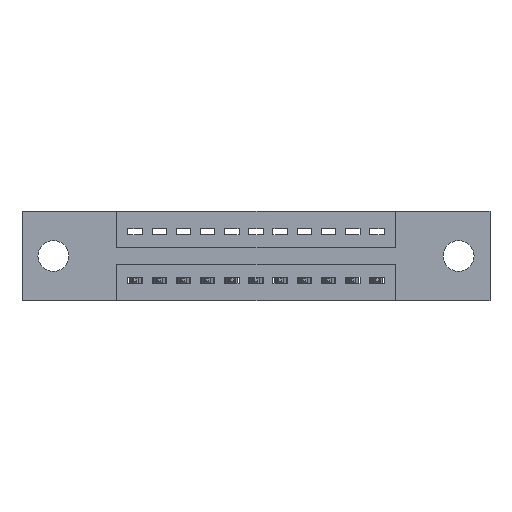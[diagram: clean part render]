
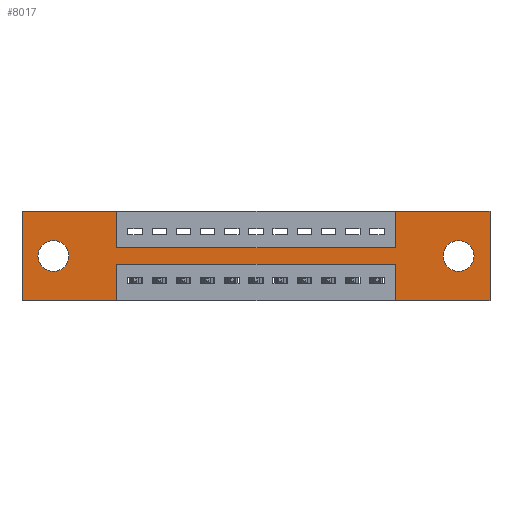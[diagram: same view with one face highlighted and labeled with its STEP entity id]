
A CAD part, front view. The second image highlights one B-rep face of the part: STEP entity #8017.
In plain terms, the highlighted planar face has unit normal (0, -1, 0).
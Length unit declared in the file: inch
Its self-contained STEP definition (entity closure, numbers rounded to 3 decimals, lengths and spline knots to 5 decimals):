
#35 = VERTEX_POINT ( 'NONE', #985 ) ;
#137 = EDGE_LOOP ( 'NONE', ( #1967, #1300 ) ) ;
#282 = EDGE_CURVE ( 'NONE', #7556, #35, #1522, .T. ) ;
#303 = EDGE_CURVE ( 'NONE', #6155, #10636, #3207, .T. ) ;
#318 = VERTEX_POINT ( 'NONE', #7704 ) ;
#332 = ORIENTED_EDGE ( 'NONE', *, *, #12484, .F. ) ;
#356 = VERTEX_POINT ( 'NONE', #3940 ) ;
#357 = VERTEX_POINT ( 'NONE', #8783 ) ;
#407 = VECTOR ( 'NONE', #10060, 39.37008 ) ;
#470 = EDGE_CURVE ( 'NONE', #2706, #356, #4051, .T. ) ;
#582 = VECTOR ( 'NONE', #11792, 39.37008 ) ;
#700 = DIRECTION ( 'NONE',  ( 0., 0., 1. ) ) ;
#711 = CARTESIAN_POINT ( 'NONE',  ( 0.13, 0., -0.185 ) ) ;
#744 = CARTESIAN_POINT ( 'NONE',  ( 0.13, 0., -0.185 ) ) ;
#775 = CARTESIAN_POINT ( 'NONE',  ( 0.3925, 0., -0.37 ) ) ;
#838 = VERTEX_POINT ( 'NONE', #2989 ) ;
#952 = ORIENTED_EDGE ( 'NONE', *, *, #10368, .F. ) ;
#960 = CARTESIAN_POINT ( 'NONE',  ( 0.3925, 0., -0.15 ) ) ;
#985 = CARTESIAN_POINT ( 'NONE',  ( 1.5425, 0., -0.15 ) ) ;
#1038 = DIRECTION ( 'NONE',  ( 1., 0., 0. ) ) ;
#1257 = VECTOR ( 'NONE', #2549, 39.37008 ) ;
#1300 = ORIENTED_EDGE ( 'NONE', *, *, #4787, .T. ) ;
#1333 = CARTESIAN_POINT ( 'NONE',  ( 0.3925, 0., 0. ) ) ;
#1406 = CARTESIAN_POINT ( 'NONE',  ( 0., 0., -0.37 ) ) ;
#1511 = DIRECTION ( 'NONE',  ( 0., 1., 0. ) ) ;
#1522 = LINE ( 'NONE', #960, #11447 ) ;
#1722 = EDGE_CURVE ( 'NONE', #357, #838, #5812, .T. ) ;
#1777 = EDGE_CURVE ( 'NONE', #7904, #7556, #3442, .T. ) ;
#1808 = LINE ( 'NONE', #6347, #7510 ) ;
#1905 = DIRECTION ( 'NONE',  ( 0., 0., -1. ) ) ;
#1967 = ORIENTED_EDGE ( 'NONE', *, *, #2109, .T. ) ;
#1987 = CARTESIAN_POINT ( 'NONE',  ( 1.805, 0., -0.185 ) ) ;
#2109 = EDGE_CURVE ( 'NONE', #2324, #10103, #3008, .T. ) ;
#2126 = ORIENTED_EDGE ( 'NONE', *, *, #6589, .F. ) ;
#2203 = AXIS2_PLACEMENT_3D ( 'NONE', #7951, #4918, #7862 ) ;
#2260 = CARTESIAN_POINT ( 'NONE',  ( 1.5425, 0., 0. ) ) ;
#2324 = VERTEX_POINT ( 'NONE', #8224 ) ;
#2549 = DIRECTION ( 'NONE',  ( -1., 0., 0. ) ) ;
#2693 = AXIS2_PLACEMENT_3D ( 'NONE', #1987, #6724, #1905 ) ;
#2706 = VERTEX_POINT ( 'NONE', #2728 ) ;
#2728 = CARTESIAN_POINT ( 'NONE',  ( 1.935, 0., 0. ) ) ;
#2920 = AXIS2_PLACEMENT_3D ( 'NONE', #1406, #9104, #11998 ) ;
#2989 = CARTESIAN_POINT ( 'NONE',  ( 1.805, 0., -0.249 ) ) ;
#3008 = CIRCLE ( 'NONE', #4929, 0.064 ) ;
#3207 = LINE ( 'NONE', #3308, #5418 ) ;
#3258 = CARTESIAN_POINT ( 'NONE',  ( 1.5425, 0., 0. ) ) ;
#3308 = CARTESIAN_POINT ( 'NONE',  ( 0., 0., -0.37 ) ) ;
#3347 = VECTOR ( 'NONE', #5261, 39.37008 ) ;
#3442 = LINE ( 'NONE', #9979, #407 ) ;
#3657 = FACE_BOUND ( 'NONE', #5722, .T. ) ;
#3702 = EDGE_CURVE ( 'NONE', #838, #357, #5535, .T. ) ;
#3780 = CARTESIAN_POINT ( 'NONE',  ( 0.3925, 0., -0.37 ) ) ;
#3822 = DIRECTION ( 'NONE',  ( -1., 0., 0. ) ) ;
#3940 = CARTESIAN_POINT ( 'NONE',  ( 1.935, 0., -0.37 ) ) ;
#4023 = VECTOR ( 'NONE', #3822, 39.37008 ) ;
#4051 = LINE ( 'NONE', #7048, #8153 ) ;
#4150 = CARTESIAN_POINT ( 'NONE',  ( 1.5425, 0., -0.22 ) ) ;
#4354 = LINE ( 'NONE', #2260, #5834 ) ;
#4513 = CARTESIAN_POINT ( 'NONE',  ( 0.3925, 0., -0.22 ) ) ;
#4698 = EDGE_LOOP ( 'NONE', ( #11630, #2126, #11438, #332, #10496, #952, #10588, #11065, #11744, #6601, #5599, #5415 ) ) ;
#4738 = DIRECTION ( 'NONE',  ( 0., 0., -1. ) ) ;
#4787 = EDGE_CURVE ( 'NONE', #10103, #2324, #12129, .T. ) ;
#4897 = VERTEX_POINT ( 'NONE', #12358 ) ;
#4918 = DIRECTION ( 'NONE',  ( 0., 1., 0. ) ) ;
#4929 = AXIS2_PLACEMENT_3D ( 'NONE', #744, #10224, #700 ) ;
#5206 = DIRECTION ( 'NONE',  ( 0., 0., -1. ) ) ;
#5261 = DIRECTION ( 'NONE',  ( 1., 0., 0. ) ) ;
#5279 = AXIS2_PLACEMENT_3D ( 'NONE', #711, #1511, #10193 ) ;
#5415 = ORIENTED_EDGE ( 'NONE', *, *, #303, .F. ) ;
#5418 = VECTOR ( 'NONE', #8992, 39.37008 ) ;
#5535 = CIRCLE ( 'NONE', #2203, 0.064 ) ;
#5599 = ORIENTED_EDGE ( 'NONE', *, *, #11273, .F. ) ;
#5672 = LINE ( 'NONE', #3780, #10332 ) ;
#5715 = VERTEX_POINT ( 'NONE', #4150 ) ;
#5722 = EDGE_LOOP ( 'NONE', ( #5741, #8024 ) ) ;
#5741 = ORIENTED_EDGE ( 'NONE', *, *, #1722, .T. ) ;
#5812 = CIRCLE ( 'NONE', #2693, 0.064 ) ;
#5834 = VECTOR ( 'NONE', #9941, 39.37008 ) ;
#6155 = VERTEX_POINT ( 'NONE', #775 ) ;
#6337 = PLANE ( 'NONE',  #2920 ) ;
#6339 = LINE ( 'NONE', #11559, #7132 ) ;
#6347 = CARTESIAN_POINT ( 'NONE',  ( 0., 0., 0. ) ) ;
#6416 = LINE ( 'NONE', #11493, #4023 ) ;
#6589 = EDGE_CURVE ( 'NONE', #5715, #4897, #7892, .T. ) ;
#6601 = ORIENTED_EDGE ( 'NONE', *, *, #6904, .F. ) ;
#6724 = DIRECTION ( 'NONE',  ( 0., 1., 0. ) ) ;
#6781 = FACE_BOUND ( 'NONE', #137, .T. ) ;
#6904 = EDGE_CURVE ( 'NONE', #318, #7904, #6339, .T. ) ;
#7048 = CARTESIAN_POINT ( 'NONE',  ( 1.935, 0., 0. ) ) ;
#7132 = VECTOR ( 'NONE', #1038, 39.37008 ) ;
#7352 = DIRECTION ( 'NONE',  ( 0., 0., 1. ) ) ;
#7510 = VECTOR ( 'NONE', #7352, 39.37008 ) ;
#7556 = VERTEX_POINT ( 'NONE', #9552 ) ;
#7704 = CARTESIAN_POINT ( 'NONE',  ( 0., 0., 0. ) ) ;
#7862 = DIRECTION ( 'NONE',  ( 0., 0., -1. ) ) ;
#7892 = LINE ( 'NONE', #4513, #1257 ) ;
#7900 = CARTESIAN_POINT ( 'NONE',  ( 1.5425, 0., -0.37 ) ) ;
#7904 = VERTEX_POINT ( 'NONE', #1333 ) ;
#7951 = CARTESIAN_POINT ( 'NONE',  ( 1.805, 0., -0.185 ) ) ;
#8017 = ADVANCED_FACE ( 'NONE', ( #3657, #6781, #12354 ), #6337, .T. ) ;
#8024 = ORIENTED_EDGE ( 'NONE', *, *, #3702, .T. ) ;
#8093 = CARTESIAN_POINT ( 'NONE',  ( 0., 0., 0. ) ) ;
#8108 = VERTEX_POINT ( 'NONE', #11007 ) ;
#8153 = VECTOR ( 'NONE', #5206, 39.37008 ) ;
#8224 = CARTESIAN_POINT ( 'NONE',  ( 0.13, 0., -0.121 ) ) ;
#8437 = LINE ( 'NONE', #7900, #582 ) ;
#8783 = CARTESIAN_POINT ( 'NONE',  ( 1.805, 0., -0.121 ) ) ;
#8992 = DIRECTION ( 'NONE',  ( -1., 0., 0. ) ) ;
#9104 = DIRECTION ( 'NONE',  ( 0., -1., 0. ) ) ;
#9552 = CARTESIAN_POINT ( 'NONE',  ( 0.3925, 0., -0.15 ) ) ;
#9941 = DIRECTION ( 'NONE',  ( 0., 0., 1. ) ) ;
#9979 = CARTESIAN_POINT ( 'NONE',  ( 0.3925, 0., 0. ) ) ;
#10060 = DIRECTION ( 'NONE',  ( 0., 0., -1. ) ) ;
#10103 = VERTEX_POINT ( 'NONE', #11268 ) ;
#10193 = DIRECTION ( 'NONE',  ( 0., 0., 1. ) ) ;
#10224 = DIRECTION ( 'NONE',  ( 0., 1., 0. ) ) ;
#10332 = VECTOR ( 'NONE', #4738, 39.37008 ) ;
#10368 = EDGE_CURVE ( 'NONE', #12074, #2706, #11449, .T. ) ;
#10496 = ORIENTED_EDGE ( 'NONE', *, *, #470, .F. ) ;
#10588 = ORIENTED_EDGE ( 'NONE', *, *, #10886, .F. ) ;
#10636 = VERTEX_POINT ( 'NONE', #12402 ) ;
#10886 = EDGE_CURVE ( 'NONE', #35, #12074, #4354, .T. ) ;
#10901 = EDGE_CURVE ( 'NONE', #8108, #5715, #8437, .T. ) ;
#11007 = CARTESIAN_POINT ( 'NONE',  ( 1.5425, 0., -0.37 ) ) ;
#11065 = ORIENTED_EDGE ( 'NONE', *, *, #282, .F. ) ;
#11268 = CARTESIAN_POINT ( 'NONE',  ( 0.13, 0., -0.249 ) ) ;
#11273 = EDGE_CURVE ( 'NONE', #10636, #318, #1808, .T. ) ;
#11438 = ORIENTED_EDGE ( 'NONE', *, *, #10901, .F. ) ;
#11447 = VECTOR ( 'NONE', #11636, 39.37008 ) ;
#11449 = LINE ( 'NONE', #8093, #3347 ) ;
#11480 = EDGE_CURVE ( 'NONE', #4897, #6155, #5672, .T. ) ;
#11493 = CARTESIAN_POINT ( 'NONE',  ( 0., 0., -0.37 ) ) ;
#11559 = CARTESIAN_POINT ( 'NONE',  ( 0., 0., 0. ) ) ;
#11630 = ORIENTED_EDGE ( 'NONE', *, *, #11480, .F. ) ;
#11636 = DIRECTION ( 'NONE',  ( 1., 0., 0. ) ) ;
#11744 = ORIENTED_EDGE ( 'NONE', *, *, #1777, .F. ) ;
#11792 = DIRECTION ( 'NONE',  ( 0., 0., 1. ) ) ;
#11998 = DIRECTION ( 'NONE',  ( 0., 0., -1. ) ) ;
#12074 = VERTEX_POINT ( 'NONE', #3258 ) ;
#12129 = CIRCLE ( 'NONE', #5279, 0.064 ) ;
#12354 = FACE_OUTER_BOUND ( 'NONE', #4698, .T. ) ;
#12358 = CARTESIAN_POINT ( 'NONE',  ( 0.3925, 0., -0.22 ) ) ;
#12402 = CARTESIAN_POINT ( 'NONE',  ( 0., 0., -0.37 ) ) ;
#12484 = EDGE_CURVE ( 'NONE', #356, #8108, #6416, .T. ) ;
